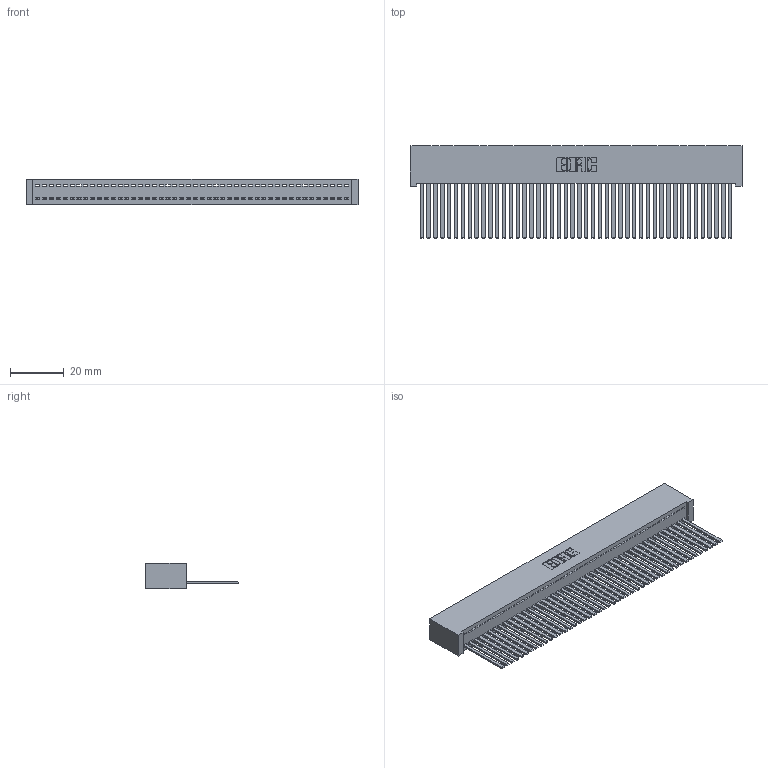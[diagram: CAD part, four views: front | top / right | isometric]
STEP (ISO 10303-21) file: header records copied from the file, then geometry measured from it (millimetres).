
FILE_DESCRIPTION (( 'STEP AP203' ), '1' );
FILE_NAME ('392-046-544-101.STEP', '2019-10-07T23:50:18', ( '' ), ( '' ), 'SwSTEP 2.0', 'SolidWorks 2016', '' );
FILE_SCHEMA (( 'CONFIG_CONTROL_DESIGN' ));
Length unit declared in the file: inch
Products named in the file (3): 342 Part_Lugless; 345-292-001_345-293-144; 392-046-544-101
Assembly tree (47 placements, depth 2):
  392-046-544-101
    342 Part_Lugless
    345-292-001_345-293-144  x46
Bounding box: 123.09 x 34.3 x 9.4 mm (x, y, z)
Volume: 11748.8 mm3; surface area: 19166.8 mm2
Topology: 47 solids, 47 shells, 2494 faces, 7543 edges, 4966 vertices
Faces by surface type: plane 1810, cylinder 684
Entity records: 27011 total; most frequent: CARTESIAN_POINT 4664, ORIENTED_EDGE 4646, DIRECTION 3915, EDGE_CURVE 2323, VECTOR 2207, LINE 2207, VERTEX_POINT 1546, AXIS2_PLACEMENT_3D 854
